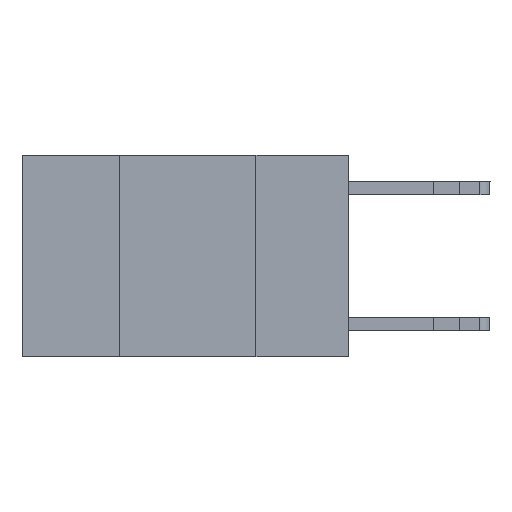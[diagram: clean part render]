
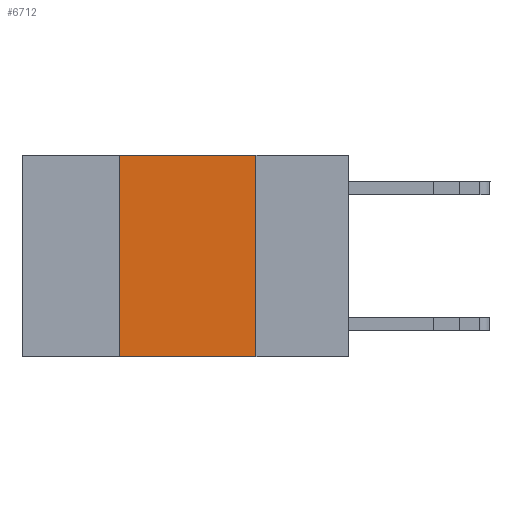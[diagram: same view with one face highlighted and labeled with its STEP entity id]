
A CAD part, left-side view. The second image highlights one B-rep face of the part: STEP entity #6712.
In plain terms, the highlighted planar face has unit normal (-1, 0, 0).
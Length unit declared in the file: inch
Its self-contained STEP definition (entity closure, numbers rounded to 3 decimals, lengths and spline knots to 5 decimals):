
#646 = EDGE_LOOP ( 'NONE', ( #12007, #15358, #2854, #11547 ) ) ;
#2854 = ORIENTED_EDGE ( 'NONE', *, *, #14735, .F. ) ;
#2965 = VECTOR ( 'NONE', #13070, 39.37008 ) ;
#3076 = CARTESIAN_POINT ( 'NONE',  ( 0., 0.6, 0. ) ) ;
#4820 = VERTEX_POINT ( 'NONE', #8280 ) ;
#4865 = DIRECTION ( 'NONE',  ( 0., -1., 0. ) ) ;
#5224 = PLANE ( 'NONE',  #13360 ) ;
#6712 = ADVANCED_FACE ( 'NONE', ( #12162 ), #5224, .F. ) ;
#7589 = LINE ( 'NONE', #11748, #2965 ) ;
#8280 = CARTESIAN_POINT ( 'NONE',  ( 0., 0.17, 0. ) ) ;
#10223 = CARTESIAN_POINT ( 'NONE',  ( 0., 0.42, 0. ) ) ;
#10412 = VERTEX_POINT ( 'NONE', #23087 ) ;
#10480 = DIRECTION ( 'NONE',  ( 0., 0., -1. ) ) ;
#11547 = ORIENTED_EDGE ( 'NONE', *, *, #12414, .T. ) ;
#11748 = CARTESIAN_POINT ( 'NONE',  ( 0., 0.17, 0. ) ) ;
#11908 = LINE ( 'NONE', #14048, #14553 ) ;
#12007 = ORIENTED_EDGE ( 'NONE', *, *, #22223, .F. ) ;
#12162 = FACE_OUTER_BOUND ( 'NONE', #646, .T. ) ;
#12380 = CARTESIAN_POINT ( 'NONE',  ( 0., 0.6, -0.37 ) ) ;
#12382 = VERTEX_POINT ( 'NONE', #19496 ) ;
#12383 = VERTEX_POINT ( 'NONE', #10223 ) ;
#12414 = EDGE_CURVE ( 'NONE', #12382, #10412, #21035, .T. ) ;
#13070 = DIRECTION ( 'NONE',  ( 0., 0., -1. ) ) ;
#13360 = AXIS2_PLACEMENT_3D ( 'NONE', #3076, #14056, #10480 ) ;
#13919 = DIRECTION ( 'NONE',  ( 0., -1., 0. ) ) ;
#13969 = VECTOR ( 'NONE', #19804, 39.37008 ) ;
#14048 = CARTESIAN_POINT ( 'NONE',  ( 0., 0.6, 0. ) ) ;
#14056 = DIRECTION ( 'NONE',  ( 1., 0., 0. ) ) ;
#14330 = CARTESIAN_POINT ( 'NONE',  ( 0., 0.42, 0. ) ) ;
#14386 = VECTOR ( 'NONE', #13919, 39.37008 ) ;
#14553 = VECTOR ( 'NONE', #4865, 39.37008 ) ;
#14735 = EDGE_CURVE ( 'NONE', #12382, #12383, #20145, .T. ) ;
#15358 = ORIENTED_EDGE ( 'NONE', *, *, #16353, .F. ) ;
#16353 = EDGE_CURVE ( 'NONE', #12383, #4820, #11908, .T. ) ;
#19496 = CARTESIAN_POINT ( 'NONE',  ( 0., 0.42, -0.37 ) ) ;
#19804 = DIRECTION ( 'NONE',  ( 0., 0., 1. ) ) ;
#20145 = LINE ( 'NONE', #14330, #13969 ) ;
#21035 = LINE ( 'NONE', #12380, #14386 ) ;
#22223 = EDGE_CURVE ( 'NONE', #4820, #10412, #7589, .T. ) ;
#23087 = CARTESIAN_POINT ( 'NONE',  ( 0., 0.17, -0.37 ) ) ;
